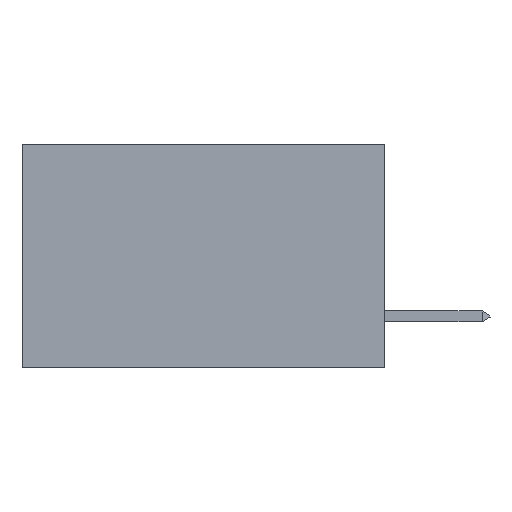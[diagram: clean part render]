
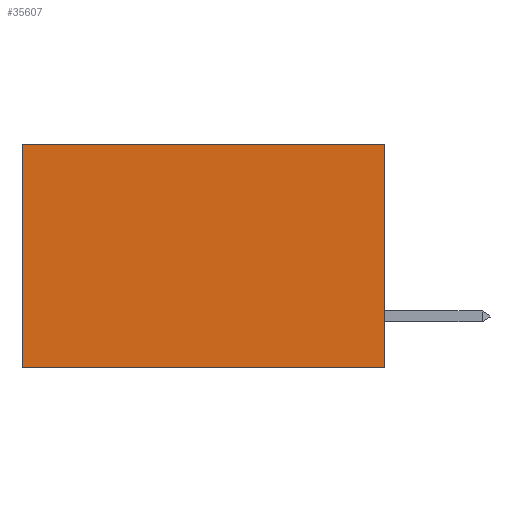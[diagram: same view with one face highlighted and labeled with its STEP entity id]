
A CAD part, left-side view. The second image highlights one B-rep face of the part: STEP entity #35607.
In plain terms, the highlighted planar face has unit normal (-1, 0, 0).
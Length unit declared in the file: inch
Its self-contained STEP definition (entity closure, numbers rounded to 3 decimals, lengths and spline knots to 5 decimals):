
#16 = VERTEX_POINT ( 'NONE', #18975 ) ;
#254 = VECTOR ( 'NONE', #20508, 39.37008 ) ;
#1605 = VERTEX_POINT ( 'NONE', #31497 ) ;
#3211 = FACE_OUTER_BOUND ( 'NONE', #34512, .T. ) ;
#4209 = AXIS2_PLACEMENT_3D ( 'NONE', #38470, #32501, #35162 ) ;
#7561 = ORIENTED_EDGE ( 'NONE', *, *, #38518, .F. ) ;
#9153 = ORIENTED_EDGE ( 'NONE', *, *, #26153, .T. ) ;
#10933 = LINE ( 'NONE', #13020, #32418 ) ;
#12891 = DIRECTION ( 'NONE',  ( 0., 1., 0. ) ) ;
#13020 = CARTESIAN_POINT ( 'NONE',  ( 0.2875, 0., -0.37 ) ) ;
#13805 = PLANE ( 'NONE',  #4209 ) ;
#15843 = VERTEX_POINT ( 'NONE', #18858 ) ;
#16173 = VERTEX_POINT ( 'NONE', #37143 ) ;
#17161 = VECTOR ( 'NONE', #19671, 39.37008 ) ;
#18858 = CARTESIAN_POINT ( 'NONE',  ( 0.2875, 0.6, -0.37 ) ) ;
#18975 = CARTESIAN_POINT ( 'NONE',  ( 0.2875, 0., -0.37 ) ) ;
#19671 = DIRECTION ( 'NONE',  ( 0., 1., 0. ) ) ;
#19691 = CARTESIAN_POINT ( 'NONE',  ( 0.2875, 0., 0. ) ) ;
#20508 = DIRECTION ( 'NONE',  ( 0., 0., -1. ) ) ;
#22118 = DIRECTION ( 'NONE',  ( 0., 0., -1. ) ) ;
#24250 = ORIENTED_EDGE ( 'NONE', *, *, #36503, .T. ) ;
#24346 = LINE ( 'NONE', #34884, #17161 ) ;
#26153 = EDGE_CURVE ( 'NONE', #16173, #1605, #24346, .T. ) ;
#26507 = ORIENTED_EDGE ( 'NONE', *, *, #35272, .F. ) ;
#27738 = VECTOR ( 'NONE', #22118, 39.37008 ) ;
#31317 = LINE ( 'NONE', #19691, #254 ) ;
#31497 = CARTESIAN_POINT ( 'NONE',  ( 0.2875, 0.6, 0. ) ) ;
#31587 = CARTESIAN_POINT ( 'NONE',  ( 0.2875, 0.6, 0. ) ) ;
#32418 = VECTOR ( 'NONE', #12891, 39.37008 ) ;
#32501 = DIRECTION ( 'NONE',  ( 1., 0., 0. ) ) ;
#34512 = EDGE_LOOP ( 'NONE', ( #24250, #26507, #7561, #9153 ) ) ;
#34884 = CARTESIAN_POINT ( 'NONE',  ( 0.2875, 0., 0. ) ) ;
#35162 = DIRECTION ( 'NONE',  ( 0., 0., -1. ) ) ;
#35272 = EDGE_CURVE ( 'NONE', #16, #15843, #10933, .T. ) ;
#35607 = ADVANCED_FACE ( 'NONE', ( #3211 ), #13805, .F. ) ;
#35804 = LINE ( 'NONE', #31587, #27738 ) ;
#36503 = EDGE_CURVE ( 'NONE', #1605, #15843, #35804, .T. ) ;
#37143 = CARTESIAN_POINT ( 'NONE',  ( 0.2875, 0., 0. ) ) ;
#38470 = CARTESIAN_POINT ( 'NONE',  ( 0.2875, 0., 0. ) ) ;
#38518 = EDGE_CURVE ( 'NONE', #16173, #16, #31317, .T. ) ;
